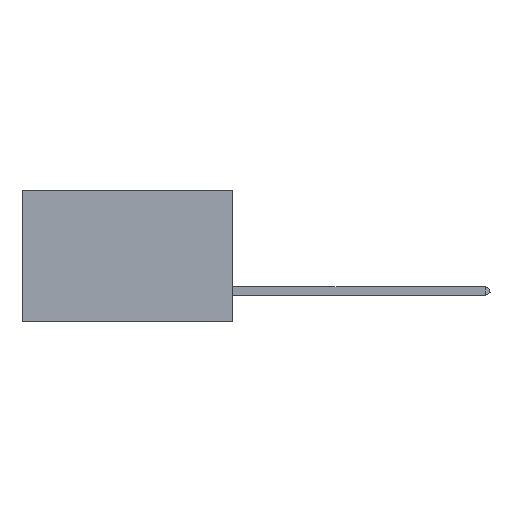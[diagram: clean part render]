
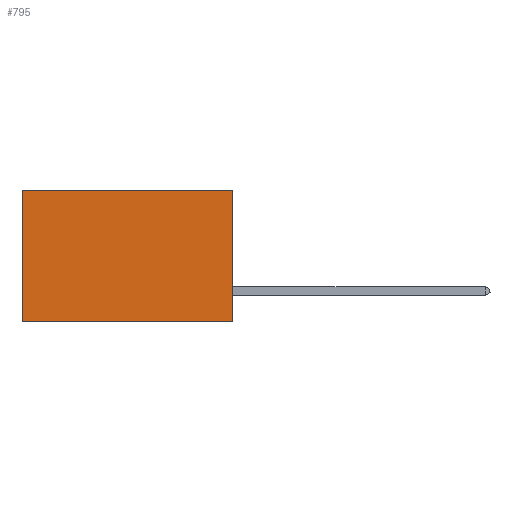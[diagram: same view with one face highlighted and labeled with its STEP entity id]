
A CAD part, left-side view. The second image highlights one B-rep face of the part: STEP entity #795.
In plain terms, the highlighted planar face has unit normal (-1, 0, 0).
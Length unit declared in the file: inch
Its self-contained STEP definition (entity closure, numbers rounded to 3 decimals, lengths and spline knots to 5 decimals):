
#738 = CARTESIAN_POINT ( 'NONE',  ( 0.2875, 0.6, -0.375 ) ) ;
#795 = ADVANCED_FACE ( 'NONE', ( #5498 ), #12963, .F. ) ;
#995 = EDGE_LOOP ( 'NONE', ( #13713, #15708, #12332, #1139 ) ) ;
#1139 = ORIENTED_EDGE ( 'NONE', *, *, #5557, .T. ) ;
#2033 = DIRECTION ( 'NONE',  ( 1., 0., 0. ) ) ;
#2423 = CARTESIAN_POINT ( 'NONE',  ( 0.2875, 0., -0.375 ) ) ;
#3796 = LINE ( 'NONE', #12527, #16487 ) ;
#3798 = CARTESIAN_POINT ( 'NONE',  ( 0.2875, 0.6, -0.375 ) ) ;
#5498 = FACE_OUTER_BOUND ( 'NONE', #995, .T. ) ;
#5557 = EDGE_CURVE ( 'NONE', #8320, #9371, #8268, .T. ) ;
#6130 = VECTOR ( 'NONE', #8948, 39.37008 ) ;
#6152 = EDGE_CURVE ( 'NONE', #9371, #13234, #12933, .T. ) ;
#6395 = CARTESIAN_POINT ( 'NONE',  ( 0.2875, 0., 0. ) ) ;
#6588 = AXIS2_PLACEMENT_3D ( 'NONE', #14160, #2033, #13027 ) ;
#7044 = DIRECTION ( 'NONE',  ( 0., 1., 0. ) ) ;
#8024 = VECTOR ( 'NONE', #9053, 39.37008 ) ;
#8268 = LINE ( 'NONE', #6395, #6130 ) ;
#8320 = VERTEX_POINT ( 'NONE', #11568 ) ;
#8948 = DIRECTION ( 'NONE',  ( 0., 1., 0. ) ) ;
#9053 = DIRECTION ( 'NONE',  ( 0., 0., -1. ) ) ;
#9371 = VERTEX_POINT ( 'NONE', #14615 ) ;
#10353 = EDGE_CURVE ( 'NONE', #13525, #13234, #3796, .T. ) ;
#11568 = CARTESIAN_POINT ( 'NONE',  ( 0.2875, 0., 0. ) ) ;
#12332 = ORIENTED_EDGE ( 'NONE', *, *, #17431, .F. ) ;
#12527 = CARTESIAN_POINT ( 'NONE',  ( 0.2875, 0., -0.375 ) ) ;
#12933 = LINE ( 'NONE', #3798, #8024 ) ;
#12963 = PLANE ( 'NONE',  #6588 ) ;
#13027 = DIRECTION ( 'NONE',  ( 0., 0., -1. ) ) ;
#13234 = VERTEX_POINT ( 'NONE', #738 ) ;
#13525 = VERTEX_POINT ( 'NONE', #2423 ) ;
#13713 = ORIENTED_EDGE ( 'NONE', *, *, #6152, .T. ) ;
#14101 = CARTESIAN_POINT ( 'NONE',  ( 0.2875, 0., -0.375 ) ) ;
#14160 = CARTESIAN_POINT ( 'NONE',  ( 0.2875, 0., -0.375 ) ) ;
#14615 = CARTESIAN_POINT ( 'NONE',  ( 0.2875, 0.6, 0. ) ) ;
#15508 = DIRECTION ( 'NONE',  ( 0., 0., -1. ) ) ;
#15708 = ORIENTED_EDGE ( 'NONE', *, *, #10353, .F. ) ;
#16413 = VECTOR ( 'NONE', #15508, 39.37008 ) ;
#16487 = VECTOR ( 'NONE', #7044, 39.37008 ) ;
#16647 = LINE ( 'NONE', #14101, #16413 ) ;
#17431 = EDGE_CURVE ( 'NONE', #8320, #13525, #16647, .T. ) ;
